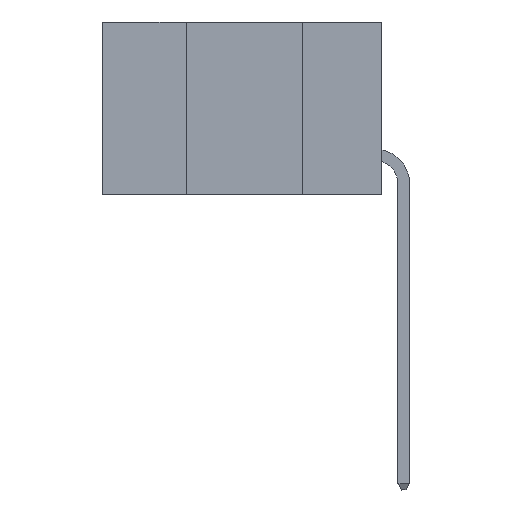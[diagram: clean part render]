
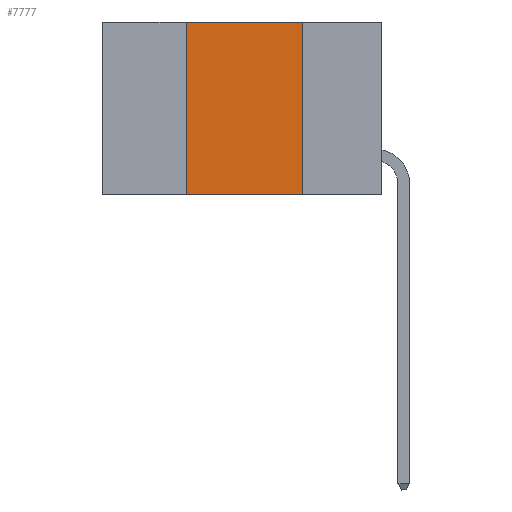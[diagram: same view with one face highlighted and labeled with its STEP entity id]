
A CAD part, left-side view. The second image highlights one B-rep face of the part: STEP entity #7777.
In plain terms, the highlighted planar face has unit normal (-1, 0, 0).
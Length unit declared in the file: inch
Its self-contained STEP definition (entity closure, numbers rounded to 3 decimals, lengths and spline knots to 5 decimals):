
#107 = EDGE_CURVE ( 'NONE', #8455, #31540, #29444, .T. ) ;
#117 = VECTOR ( 'NONE', #29394, 39.37008 ) ;
#1769 = CARTESIAN_POINT ( 'NONE',  ( 0., 0.6, 0. ) ) ;
#2498 = CARTESIAN_POINT ( 'NONE',  ( 0., 0.17, 0. ) ) ;
#2802 = VECTOR ( 'NONE', #9445, 39.37008 ) ;
#4504 = PLANE ( 'NONE',  #8080 ) ;
#6146 = ORIENTED_EDGE ( 'NONE', *, *, #107, .F. ) ;
#7625 = DIRECTION ( 'NONE',  ( 0., 0., -1. ) ) ;
#7777 = ADVANCED_FACE ( 'NONE', ( #12538 ), #4504, .F. ) ;
#8013 = DIRECTION ( 'NONE',  ( 1., 0., 0. ) ) ;
#8080 = AXIS2_PLACEMENT_3D ( 'NONE', #1769, #8013, #7625 ) ;
#8455 = VERTEX_POINT ( 'NONE', #18508 ) ;
#8562 = ORIENTED_EDGE ( 'NONE', *, *, #27051, .T. ) ;
#9445 = DIRECTION ( 'NONE',  ( 0., 0., 1. ) ) ;
#9448 = ORIENTED_EDGE ( 'NONE', *, *, #27345, .F. ) ;
#9660 = DIRECTION ( 'NONE',  ( 0., -1., 0. ) ) ;
#12538 = FACE_OUTER_BOUND ( 'NONE', #20907, .T. ) ;
#13245 = ORIENTED_EDGE ( 'NONE', *, *, #22216, .F. ) ;
#13968 = VECTOR ( 'NONE', #24380, 39.37008 ) ;
#14901 = LINE ( 'NONE', #18687, #13968 ) ;
#15108 = VECTOR ( 'NONE', #9660, 39.37008 ) ;
#15141 = VERTEX_POINT ( 'NONE', #29187 ) ;
#16064 = LINE ( 'NONE', #16534, #15108 ) ;
#16534 = CARTESIAN_POINT ( 'NONE',  ( 0., 0.6, -0.37 ) ) ;
#16984 = LINE ( 'NONE', #2498, #117 ) ;
#17299 = CARTESIAN_POINT ( 'NONE',  ( 0., 0.17, -0.37 ) ) ;
#18508 = CARTESIAN_POINT ( 'NONE',  ( 0., 0.42, -0.37 ) ) ;
#18687 = CARTESIAN_POINT ( 'NONE',  ( 0., 0.6, 0. ) ) ;
#20903 = CARTESIAN_POINT ( 'NONE',  ( 0., 0.42, 0. ) ) ;
#20907 = EDGE_LOOP ( 'NONE', ( #9448, #13245, #6146, #8562 ) ) ;
#22216 = EDGE_CURVE ( 'NONE', #31540, #15141, #14901, .T. ) ;
#24380 = DIRECTION ( 'NONE',  ( 0., -1., 0. ) ) ;
#27051 = EDGE_CURVE ( 'NONE', #8455, #36015, #16064, .T. ) ;
#27345 = EDGE_CURVE ( 'NONE', #15141, #36015, #16984, .T. ) ;
#29187 = CARTESIAN_POINT ( 'NONE',  ( 0., 0.17, 0. ) ) ;
#29394 = DIRECTION ( 'NONE',  ( 0., 0., -1. ) ) ;
#29444 = LINE ( 'NONE', #29679, #2802 ) ;
#29679 = CARTESIAN_POINT ( 'NONE',  ( 0., 0.42, 0. ) ) ;
#31540 = VERTEX_POINT ( 'NONE', #20903 ) ;
#36015 = VERTEX_POINT ( 'NONE', #17299 ) ;
